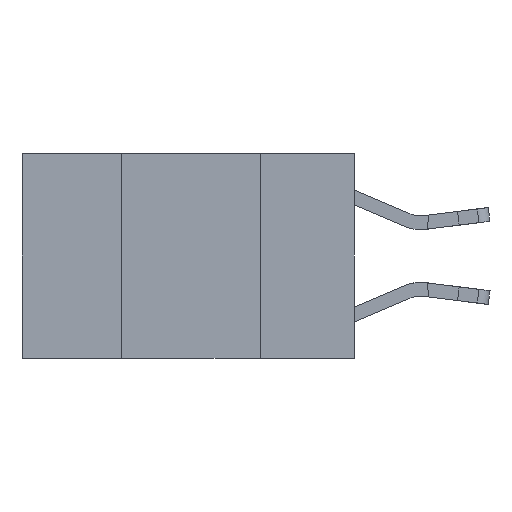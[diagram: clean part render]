
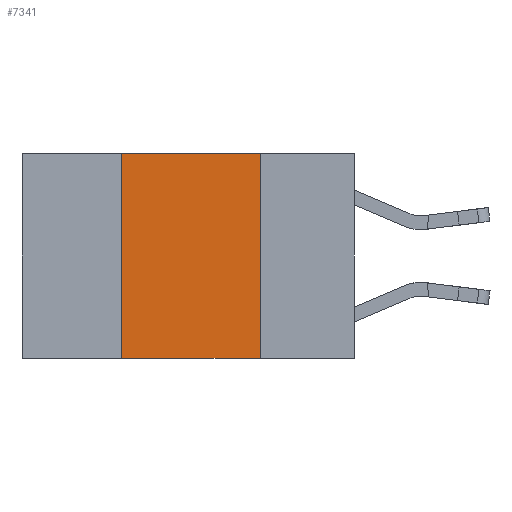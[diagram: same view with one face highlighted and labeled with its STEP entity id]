
A CAD part, left-side view. The second image highlights one B-rep face of the part: STEP entity #7341.
In plain terms, the highlighted planar face has unit normal (-1, 0, 0).
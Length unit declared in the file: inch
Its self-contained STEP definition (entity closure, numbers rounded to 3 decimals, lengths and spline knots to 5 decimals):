
#326 = VERTEX_POINT ( 'NONE', #2704 ) ;
#1275 = VECTOR ( 'NONE', #10190, 39.37008 ) ;
#1709 = ORIENTED_EDGE ( 'NONE', *, *, #5124, .F. ) ;
#2704 = CARTESIAN_POINT ( 'NONE',  ( 0., 0.17, -0.37 ) ) ;
#2744 = PLANE ( 'NONE',  #5246 ) ;
#2905 = EDGE_CURVE ( 'NONE', #5925, #326, #14582, .T. ) ;
#2947 = EDGE_CURVE ( 'NONE', #13521, #6085, #10793, .T. ) ;
#2964 = EDGE_CURVE ( 'NONE', #13521, #326, #4376, .T. ) ;
#3622 = FACE_OUTER_BOUND ( 'NONE', #14480, .T. ) ;
#3795 = CARTESIAN_POINT ( 'NONE',  ( 0., 0.42, 0. ) ) ;
#3915 = CARTESIAN_POINT ( 'NONE',  ( 0., 0.6, 0. ) ) ;
#4376 = LINE ( 'NONE', #14931, #1275 ) ;
#4498 = LINE ( 'NONE', #7908, #7155 ) ;
#5067 = DIRECTION ( 'NONE',  ( 1., 0., 0. ) ) ;
#5124 = EDGE_CURVE ( 'NONE', #6085, #5925, #4498, .T. ) ;
#5246 = AXIS2_PLACEMENT_3D ( 'NONE', #3915, #5067, #13021 ) ;
#5668 = DIRECTION ( 'NONE',  ( 0., -1., 0. ) ) ;
#5857 = CARTESIAN_POINT ( 'NONE',  ( 0., 0.17, 0. ) ) ;
#5925 = VERTEX_POINT ( 'NONE', #12770 ) ;
#6085 = VERTEX_POINT ( 'NONE', #3795 ) ;
#6276 = CARTESIAN_POINT ( 'NONE',  ( 0., 0.42, 0. ) ) ;
#7155 = VECTOR ( 'NONE', #5668, 39.37008 ) ;
#7341 = ADVANCED_FACE ( 'NONE', ( #3622 ), #2744, .F. ) ;
#7704 = DIRECTION ( 'NONE',  ( 0., 0., 1. ) ) ;
#7908 = CARTESIAN_POINT ( 'NONE',  ( 0., 0.6, 0. ) ) ;
#8014 = ORIENTED_EDGE ( 'NONE', *, *, #2905, .F. ) ;
#10190 = DIRECTION ( 'NONE',  ( 0., -1., 0. ) ) ;
#10793 = LINE ( 'NONE', #6276, #13485 ) ;
#10859 = DIRECTION ( 'NONE',  ( 0., 0., -1. ) ) ;
#11371 = ORIENTED_EDGE ( 'NONE', *, *, #2947, .F. ) ;
#12243 = CARTESIAN_POINT ( 'NONE',  ( 0., 0.42, -0.37 ) ) ;
#12770 = CARTESIAN_POINT ( 'NONE',  ( 0., 0.17, 0. ) ) ;
#13021 = DIRECTION ( 'NONE',  ( 0., 0., -1. ) ) ;
#13485 = VECTOR ( 'NONE', #7704, 39.37008 ) ;
#13521 = VERTEX_POINT ( 'NONE', #12243 ) ;
#14196 = VECTOR ( 'NONE', #10859, 39.37008 ) ;
#14456 = ORIENTED_EDGE ( 'NONE', *, *, #2964, .T. ) ;
#14480 = EDGE_LOOP ( 'NONE', ( #8014, #1709, #11371, #14456 ) ) ;
#14582 = LINE ( 'NONE', #5857, #14196 ) ;
#14931 = CARTESIAN_POINT ( 'NONE',  ( 0., 0.6, -0.37 ) ) ;
